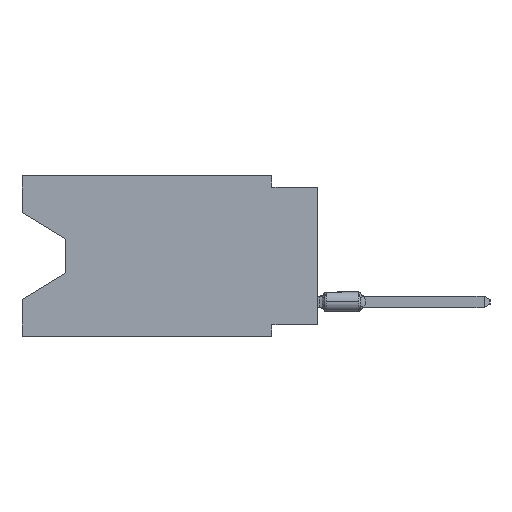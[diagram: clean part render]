
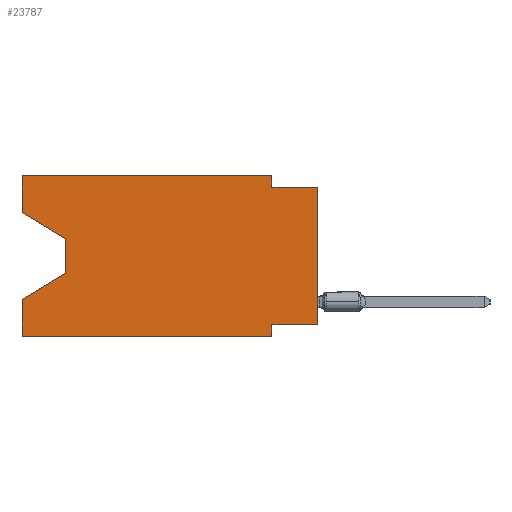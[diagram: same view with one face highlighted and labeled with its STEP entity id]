
A CAD part, left-side view. The second image highlights one B-rep face of the part: STEP entity #23787.
In plain terms, the highlighted planar face has unit normal (-1, 0, 0).
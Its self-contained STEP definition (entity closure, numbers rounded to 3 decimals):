
#45 = CARTESIAN_POINT ( 'NONE',  ( 0., 16.383, -2.038 ) ) ;
#317 = VECTOR ( 'NONE', #4376, 1000. ) ;
#477 = VERTEX_POINT ( 'NONE', #11366 ) ;
#757 = VERTEX_POINT ( 'NONE', #23203 ) ;
#1278 = CARTESIAN_POINT ( 'NONE',  ( 0., 0., -0.635 ) ) ;
#1353 = ORIENTED_EDGE ( 'NONE', *, *, #22623, .T. ) ;
#1414 = CARTESIAN_POINT ( 'NONE',  ( 0., 0., -0.635 ) ) ;
#1569 = VECTOR ( 'NONE', #4480, 1000. ) ;
#1585 = EDGE_CURVE ( 'NONE', #7368, #477, #18520, .T. ) ;
#1646 = LINE ( 'NONE', #15973, #18634 ) ;
#1843 = VERTEX_POINT ( 'NONE', #16862 ) ;
#2030 = CARTESIAN_POINT ( 'NONE',  ( 0., 0., -8.255 ) ) ;
#2204 = VECTOR ( 'NONE', #4630, 1000. ) ;
#2276 = CARTESIAN_POINT ( 'NONE',  ( 0., 13.97, -5.385 ) ) ;
#2831 = DIRECTION ( 'NONE',  ( 0., 0.855, -0.519 ) ) ;
#3357 = VECTOR ( 'NONE', #2831, 1000. ) ;
#3876 = LINE ( 'NONE', #27620, #13729 ) ;
#3979 = EDGE_CURVE ( 'NONE', #9795, #757, #30251, .T. ) ;
#4376 = DIRECTION ( 'NONE',  ( 0., 0., -1. ) ) ;
#4480 = DIRECTION ( 'NONE',  ( 0., 0., 1. ) ) ;
#4630 = DIRECTION ( 'NONE',  ( 0., -0.855, -0.519 ) ) ;
#4825 = VERTEX_POINT ( 'NONE', #25503 ) ;
#5026 = CARTESIAN_POINT ( 'NONE',  ( 0., 0., 0. ) ) ;
#5954 = EDGE_CURVE ( 'NONE', #16488, #12450, #23004, .T. ) ;
#6179 = ORIENTED_EDGE ( 'NONE', *, *, #24273, .F. ) ;
#6530 = CARTESIAN_POINT ( 'NONE',  ( 0., 2.54, -8.89 ) ) ;
#6695 = VERTEX_POINT ( 'NONE', #26482 ) ;
#6701 = CARTESIAN_POINT ( 'NONE',  ( 0., 2.54, 0. ) ) ;
#7368 = VERTEX_POINT ( 'NONE', #2030 ) ;
#7576 = ORIENTED_EDGE ( 'NONE', *, *, #16179, .F. ) ;
#7795 = VECTOR ( 'NONE', #23865, 1000. ) ;
#8878 = DIRECTION ( 'NONE',  ( 0., 0., 1. ) ) ;
#8969 = VERTEX_POINT ( 'NONE', #22636 ) ;
#9566 = EDGE_CURVE ( 'NONE', #1843, #8969, #13081, .T. ) ;
#9741 = VERTEX_POINT ( 'NONE', #21484 ) ;
#9795 = VERTEX_POINT ( 'NONE', #45 ) ;
#10989 = DIRECTION ( 'NONE',  ( 0., -1., 0. ) ) ;
#11366 = CARTESIAN_POINT ( 'NONE',  ( 0., 2.54, -8.255 ) ) ;
#11506 = ORIENTED_EDGE ( 'NONE', *, *, #13521, .T. ) ;
#11631 = CARTESIAN_POINT ( 'NONE',  ( 0., 16.383, -8.89 ) ) ;
#11742 = CARTESIAN_POINT ( 'NONE',  ( 0., 16.383, -2.038 ) ) ;
#12227 = DIRECTION ( 'NONE',  ( 0., 0., -1. ) ) ;
#12450 = VERTEX_POINT ( 'NONE', #1414 ) ;
#13081 = LINE ( 'NONE', #11631, #29083 ) ;
#13142 = DIRECTION ( 'NONE',  ( 0., 0., -1. ) ) ;
#13210 = AXIS2_PLACEMENT_3D ( 'NONE', #29189, #28724, #12227 ) ;
#13240 = ORIENTED_EDGE ( 'NONE', *, *, #5954, .F. ) ;
#13521 = EDGE_CURVE ( 'NONE', #7368, #12450, #24167, .T. ) ;
#13729 = VECTOR ( 'NONE', #13142, 1000. ) ;
#13730 = EDGE_CURVE ( 'NONE', #4825, #6695, #1646, .T. ) ;
#15134 = VECTOR ( 'NONE', #8878, 1000. ) ;
#15973 = CARTESIAN_POINT ( 'NONE',  ( 0., 16.383, 0. ) ) ;
#15988 = ORIENTED_EDGE ( 'NONE', *, *, #9566, .T. ) ;
#16124 = DIRECTION ( 'NONE',  ( 0., -1., 0. ) ) ;
#16179 = EDGE_CURVE ( 'NONE', #477, #8969, #25506, .T. ) ;
#16200 = LINE ( 'NONE', #25609, #1569 ) ;
#16210 = CARTESIAN_POINT ( 'NONE',  ( 0., 0., -8.255 ) ) ;
#16488 = VERTEX_POINT ( 'NONE', #17889 ) ;
#16838 = FACE_OUTER_BOUND ( 'NONE', #19989, .T. ) ;
#16862 = CARTESIAN_POINT ( 'NONE',  ( 0., 16.383, -8.89 ) ) ;
#17150 = VECTOR ( 'NONE', #29721, 1000. ) ;
#17889 = CARTESIAN_POINT ( 'NONE',  ( 0., 2.54, -0.635 ) ) ;
#18278 = LINE ( 'NONE', #20454, #15134 ) ;
#18520 = LINE ( 'NONE', #16210, #28680 ) ;
#18634 = VECTOR ( 'NONE', #16124, 1000. ) ;
#18706 = LINE ( 'NONE', #28585, #3357 ) ;
#18786 = EDGE_CURVE ( 'NONE', #757, #19692, #3876, .T. ) ;
#19461 = PLANE ( 'NONE',  #13210 ) ;
#19692 = VERTEX_POINT ( 'NONE', #2276 ) ;
#19989 = EDGE_LOOP ( 'NONE', ( #25109, #28631, #1353, #28721, #15988, #7576, #26392, #11506, #13240, #6179, #21830, #20926 ) ) ;
#20304 = LINE ( 'NONE', #6701, #17150 ) ;
#20454 = CARTESIAN_POINT ( 'NONE',  ( 0., 16.383, 0. ) ) ;
#20908 = VECTOR ( 'NONE', #10989, 1000. ) ;
#20926 = ORIENTED_EDGE ( 'NONE', *, *, #23068, .F. ) ;
#21484 = CARTESIAN_POINT ( 'NONE',  ( 0., 16.383, -6.852 ) ) ;
#21830 = ORIENTED_EDGE ( 'NONE', *, *, #13730, .F. ) ;
#22073 = DIRECTION ( 'NONE',  ( 0., 1., 0. ) ) ;
#22623 = EDGE_CURVE ( 'NONE', #19692, #9741, #18706, .T. ) ;
#22636 = CARTESIAN_POINT ( 'NONE',  ( 0., 2.54, -8.89 ) ) ;
#23004 = LINE ( 'NONE', #1278, #20908 ) ;
#23068 = EDGE_CURVE ( 'NONE', #9795, #4825, #18278, .T. ) ;
#23203 = CARTESIAN_POINT ( 'NONE',  ( 0., 13.97, -3.505 ) ) ;
#23787 = ADVANCED_FACE ( 'NONE', ( #16838 ), #19461, .F. ) ;
#23865 = DIRECTION ( 'NONE',  ( 0., 0., 1. ) ) ;
#24167 = LINE ( 'NONE', #5026, #7795 ) ;
#24273 = EDGE_CURVE ( 'NONE', #6695, #16488, #20304, .T. ) ;
#25109 = ORIENTED_EDGE ( 'NONE', *, *, #3979, .T. ) ;
#25320 = EDGE_CURVE ( 'NONE', #1843, #9741, #16200, .T. ) ;
#25503 = CARTESIAN_POINT ( 'NONE',  ( 0., 16.383, 0. ) ) ;
#25506 = LINE ( 'NONE', #6530, #317 ) ;
#25609 = CARTESIAN_POINT ( 'NONE',  ( 0., 16.383, 0. ) ) ;
#26392 = ORIENTED_EDGE ( 'NONE', *, *, #1585, .F. ) ;
#26482 = CARTESIAN_POINT ( 'NONE',  ( 0., 2.54, 0. ) ) ;
#27620 = CARTESIAN_POINT ( 'NONE',  ( 0., 13.97, -3.505 ) ) ;
#27824 = DIRECTION ( 'NONE',  ( 0., -1., 0. ) ) ;
#28585 = CARTESIAN_POINT ( 'NONE',  ( 0., 13.97, -5.385 ) ) ;
#28631 = ORIENTED_EDGE ( 'NONE', *, *, #18786, .T. ) ;
#28680 = VECTOR ( 'NONE', #22073, 1000. ) ;
#28721 = ORIENTED_EDGE ( 'NONE', *, *, #25320, .F. ) ;
#28724 = DIRECTION ( 'NONE',  ( 1., 0., 0. ) ) ;
#29083 = VECTOR ( 'NONE', #27824, 1000. ) ;
#29189 = CARTESIAN_POINT ( 'NONE',  ( 0., 16.383, 0. ) ) ;
#29721 = DIRECTION ( 'NONE',  ( 0., 0., -1. ) ) ;
#30251 = LINE ( 'NONE', #11742, #2204 ) ;
